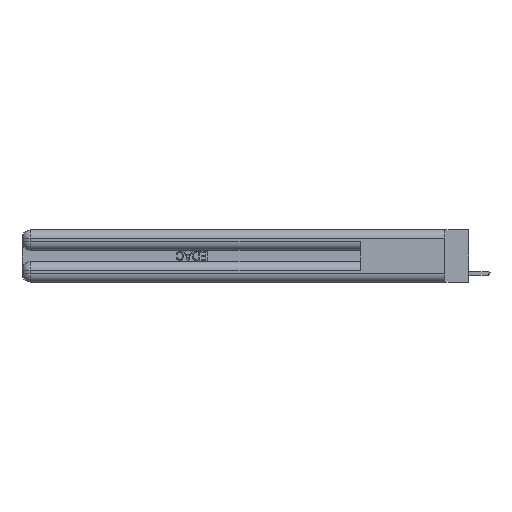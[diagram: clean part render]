
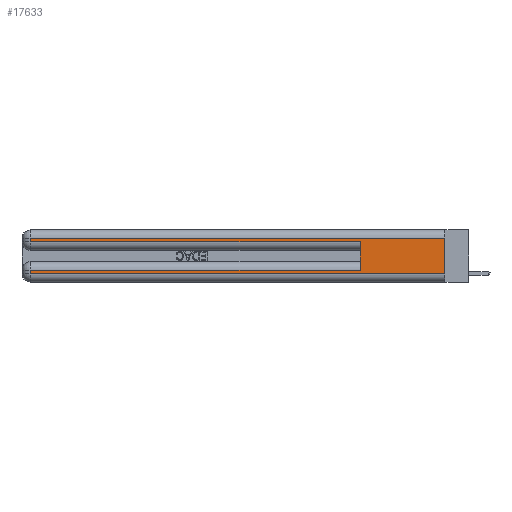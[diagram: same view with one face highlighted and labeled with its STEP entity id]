
A CAD part, left-side view. The second image highlights one B-rep face of the part: STEP entity #17633.
In plain terms, the highlighted planar face has unit normal (-1, 0, 0).
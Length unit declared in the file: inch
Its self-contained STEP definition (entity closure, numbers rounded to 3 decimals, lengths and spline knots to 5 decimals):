
#641 = VECTOR ( 'NONE', #13331, 39.37008 ) ;
#950 = EDGE_CURVE ( 'NONE', #28227, #15575, #28831, .T. ) ;
#1013 = ORIENTED_EDGE ( 'NONE', *, *, #950, .T. ) ;
#1043 = ORIENTED_EDGE ( 'NONE', *, *, #14454, .F. ) ;
#1107 = CARTESIAN_POINT ( 'NONE',  ( 0., 2.94, 0.37 ) ) ;
#2020 = LINE ( 'NONE', #31079, #28978 ) ;
#2485 = CARTESIAN_POINT ( 'NONE',  ( 0., 2.94, 0.06 ) ) ;
#2505 = DIRECTION ( 'NONE',  ( 0., 0., -1. ) ) ;
#2575 = EDGE_CURVE ( 'NONE', #14744, #28227, #7117, .T. ) ;
#2697 = VECTOR ( 'NONE', #6946, 39.37008 ) ;
#2810 = CARTESIAN_POINT ( 'NONE',  ( 0., 2.94, 0.285 ) ) ;
#6443 = ORIENTED_EDGE ( 'NONE', *, *, #20484, .T. ) ;
#6946 = DIRECTION ( 'NONE',  ( 0., 0., 1. ) ) ;
#7116 = CARTESIAN_POINT ( 'NONE',  ( 0., 2.94, 0.37 ) ) ;
#7117 = LINE ( 'NONE', #30505, #641 ) ;
#7347 = CARTESIAN_POINT ( 'NONE',  ( 0., 0., 0.31 ) ) ;
#7443 = VERTEX_POINT ( 'NONE', #2810 ) ;
#10768 = AXIS2_PLACEMENT_3D ( 'NONE', #20968, #20868, #21375 ) ;
#10940 = ORIENTED_EDGE ( 'NONE', *, *, #26989, .F. ) ;
#11584 = CARTESIAN_POINT ( 'NONE',  ( 0., 0.6, 0.145 ) ) ;
#11640 = DIRECTION ( 'NONE',  ( 0., 1., 0. ) ) ;
#11970 = DIRECTION ( 'NONE',  ( 0., -1., 0. ) ) ;
#12881 = DIRECTION ( 'NONE',  ( 0., -1., 0. ) ) ;
#13020 = VECTOR ( 'NONE', #14725, 39.37008 ) ;
#13331 = DIRECTION ( 'NONE',  ( 0., 1., 0. ) ) ;
#13482 = EDGE_LOOP ( 'NONE', ( #1043, #14948, #19260, #31737, #10940, #13559, #1013, #6443 ) ) ;
#13559 = ORIENTED_EDGE ( 'NONE', *, *, #2575, .T. ) ;
#13825 = EDGE_CURVE ( 'NONE', #7443, #26944, #21137, .T. ) ;
#14454 = EDGE_CURVE ( 'NONE', #25339, #22996, #23773, .T. ) ;
#14725 = DIRECTION ( 'NONE',  ( 0., 0., -1. ) ) ;
#14744 = VERTEX_POINT ( 'NONE', #28317 ) ;
#14948 = ORIENTED_EDGE ( 'NONE', *, *, #16146, .T. ) ;
#15000 = CARTESIAN_POINT ( 'NONE',  ( 0., 0., 0.37 ) ) ;
#15575 = VERTEX_POINT ( 'NONE', #2485 ) ;
#16146 = EDGE_CURVE ( 'NONE', #25339, #26511, #2020, .T. ) ;
#17244 = FACE_OUTER_BOUND ( 'NONE', #13482, .T. ) ;
#17633 = ADVANCED_FACE ( 'NONE', ( #17244 ), #25704, .F. ) ;
#18641 = DIRECTION ( 'NONE',  ( 0., 0., -1. ) ) ;
#18782 = LINE ( 'NONE', #11584, #2697 ) ;
#19260 = ORIENTED_EDGE ( 'NONE', *, *, #30399, .T. ) ;
#19402 = LINE ( 'NONE', #24932, #27963 ) ;
#19667 = CARTESIAN_POINT ( 'NONE',  ( 0., 2.94, 0.085 ) ) ;
#20484 = EDGE_CURVE ( 'NONE', #15575, #22996, #19402, .T. ) ;
#20737 = VECTOR ( 'NONE', #11970, 39.37008 ) ;
#20868 = DIRECTION ( 'NONE',  ( 1., 0., 0. ) ) ;
#20968 = CARTESIAN_POINT ( 'NONE',  ( 0., 0., 0.37 ) ) ;
#21137 = LINE ( 'NONE', #31800, #20737 ) ;
#21375 = DIRECTION ( 'NONE',  ( 0., 0., -1. ) ) ;
#22606 = VECTOR ( 'NONE', #2505, 39.37008 ) ;
#22996 = VERTEX_POINT ( 'NONE', #31133 ) ;
#23773 = LINE ( 'NONE', #15000, #22606 ) ;
#24932 = CARTESIAN_POINT ( 'NONE',  ( 0., 0., 0.06 ) ) ;
#25339 = VERTEX_POINT ( 'NONE', #7347 ) ;
#25704 = PLANE ( 'NONE',  #10768 ) ;
#26312 = CARTESIAN_POINT ( 'NONE',  ( 0., 0.6, 0.285 ) ) ;
#26511 = VERTEX_POINT ( 'NONE', #30052 ) ;
#26944 = VERTEX_POINT ( 'NONE', #26312 ) ;
#26989 = EDGE_CURVE ( 'NONE', #14744, #26944, #18782, .T. ) ;
#27963 = VECTOR ( 'NONE', #12881, 39.37008 ) ;
#28227 = VERTEX_POINT ( 'NONE', #19667 ) ;
#28317 = CARTESIAN_POINT ( 'NONE',  ( 0., 0.6, 0.085 ) ) ;
#28633 = LINE ( 'NONE', #1107, #29407 ) ;
#28831 = LINE ( 'NONE', #7116, #13020 ) ;
#28978 = VECTOR ( 'NONE', #11640, 39.37008 ) ;
#29407 = VECTOR ( 'NONE', #18641, 39.37008 ) ;
#30052 = CARTESIAN_POINT ( 'NONE',  ( 0., 2.94, 0.31 ) ) ;
#30399 = EDGE_CURVE ( 'NONE', #26511, #7443, #28633, .T. ) ;
#30505 = CARTESIAN_POINT ( 'NONE',  ( 0., 0., 0.085 ) ) ;
#31079 = CARTESIAN_POINT ( 'NONE',  ( 0., 0., 0.31 ) ) ;
#31133 = CARTESIAN_POINT ( 'NONE',  ( 0., 0., 0.06 ) ) ;
#31737 = ORIENTED_EDGE ( 'NONE', *, *, #13825, .T. ) ;
#31800 = CARTESIAN_POINT ( 'NONE',  ( 0., 0., 0.285 ) ) ;
